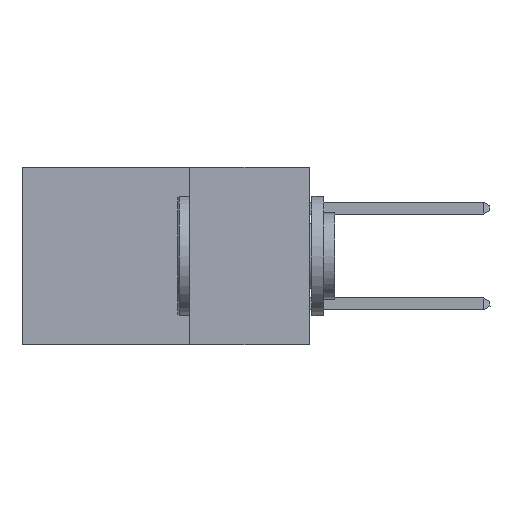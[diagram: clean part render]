
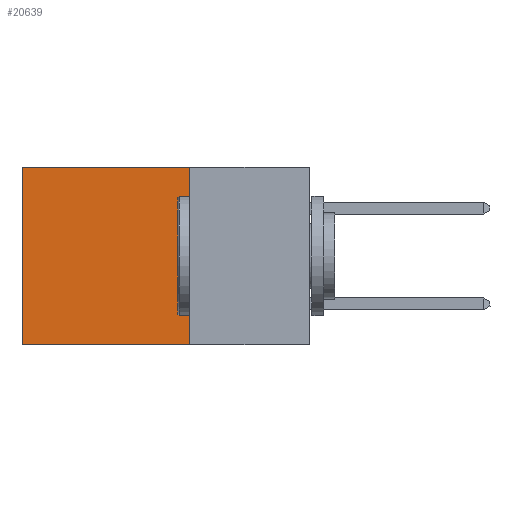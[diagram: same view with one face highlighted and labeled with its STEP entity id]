
A CAD part, left-side view. The second image highlights one B-rep face of the part: STEP entity #20639.
In plain terms, the highlighted planar face has unit normal (-1, 0, 0).
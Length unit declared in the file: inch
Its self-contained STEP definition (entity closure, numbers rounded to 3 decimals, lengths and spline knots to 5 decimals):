
#447 = CARTESIAN_POINT ( 'NONE',  ( 0.2875, 0.6, 0. ) ) ;
#672 = CARTESIAN_POINT ( 'NONE',  ( 0.2875, 0.25, -0.37 ) ) ;
#1317 = DIRECTION ( 'NONE',  ( 0., 0., -1. ) ) ;
#1473 = CARTESIAN_POINT ( 'NONE',  ( 0.2875, 0.25, -0.37 ) ) ;
#1897 = VERTEX_POINT ( 'NONE', #447 ) ;
#2066 = DIRECTION ( 'NONE',  ( 0., 0., -1. ) ) ;
#2308 = LINE ( 'NONE', #15911, #7084 ) ;
#3622 = CARTESIAN_POINT ( 'NONE',  ( 0.2875, 0.25, 0. ) ) ;
#4152 = DIRECTION ( 'NONE',  ( 0., 1., 0. ) ) ;
#4572 = EDGE_LOOP ( 'NONE', ( #8079, #20154, #15419, #21855 ) ) ;
#5218 = EDGE_CURVE ( 'NONE', #1897, #5627, #13677, .T. ) ;
#5273 = LINE ( 'NONE', #17484, #9885 ) ;
#5627 = VERTEX_POINT ( 'NONE', #20472 ) ;
#6640 = EDGE_CURVE ( 'NONE', #7619, #5627, #16013, .T. ) ;
#6988 = VECTOR ( 'NONE', #4152, 39.37008 ) ;
#7084 = VECTOR ( 'NONE', #2066, 39.37008 ) ;
#7619 = VERTEX_POINT ( 'NONE', #1473 ) ;
#8079 = ORIENTED_EDGE ( 'NONE', *, *, #5218, .T. ) ;
#9885 = VECTOR ( 'NONE', #19242, 39.37008 ) ;
#10084 = PLANE ( 'NONE',  #22465 ) ;
#11782 = DIRECTION ( 'NONE',  ( 1., 0., 0. ) ) ;
#12938 = DIRECTION ( 'NONE',  ( 0., 0., -1. ) ) ;
#13677 = LINE ( 'NONE', #19766, #22278 ) ;
#15419 = ORIENTED_EDGE ( 'NONE', *, *, #15979, .F. ) ;
#15911 = CARTESIAN_POINT ( 'NONE',  ( 0.2875, 0.25, 0. ) ) ;
#15922 = FACE_OUTER_BOUND ( 'NONE', #4572, .T. ) ;
#15979 = EDGE_CURVE ( 'NONE', #18239, #7619, #2308, .T. ) ;
#16013 = LINE ( 'NONE', #672, #6988 ) ;
#17484 = CARTESIAN_POINT ( 'NONE',  ( 0.2875, 0.25, 0. ) ) ;
#18239 = VERTEX_POINT ( 'NONE', #3622 ) ;
#19242 = DIRECTION ( 'NONE',  ( 0., 1., 0. ) ) ;
#19766 = CARTESIAN_POINT ( 'NONE',  ( 0.2875, 0.6, 0. ) ) ;
#20154 = ORIENTED_EDGE ( 'NONE', *, *, #6640, .F. ) ;
#20472 = CARTESIAN_POINT ( 'NONE',  ( 0.2875, 0.6, -0.37 ) ) ;
#20639 = ADVANCED_FACE ( 'NONE', ( #15922 ), #10084, .F. ) ;
#20887 = EDGE_CURVE ( 'NONE', #18239, #1897, #5273, .T. ) ;
#21855 = ORIENTED_EDGE ( 'NONE', *, *, #20887, .T. ) ;
#22018 = CARTESIAN_POINT ( 'NONE',  ( 0.2875, 0.25, 0. ) ) ;
#22278 = VECTOR ( 'NONE', #12938, 39.37008 ) ;
#22465 = AXIS2_PLACEMENT_3D ( 'NONE', #22018, #11782, #1317 ) ;
